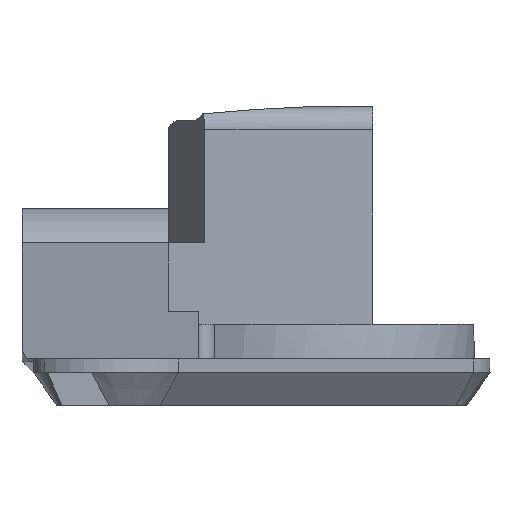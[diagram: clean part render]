
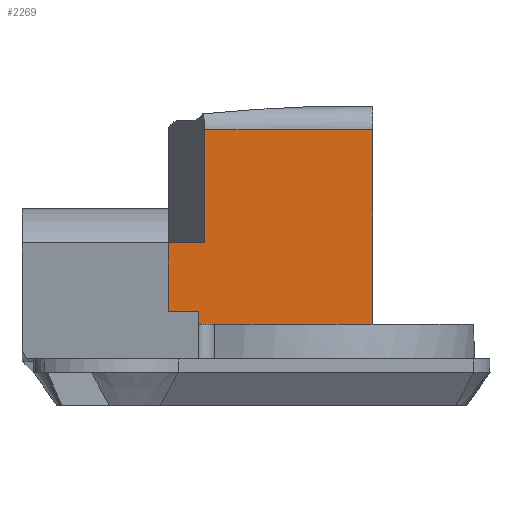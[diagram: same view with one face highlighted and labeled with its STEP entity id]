
A CAD part, left-side view. The second image highlights one B-rep face of the part: STEP entity #2269.
In plain terms, the highlighted planar face has unit normal (-1, 0, 0).
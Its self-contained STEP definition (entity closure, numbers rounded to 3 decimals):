
#254=FACE_OUTER_BOUND('',#388,.T.);
#388=EDGE_LOOP('',(#1855,#1856,#1857,#1858,#1859,#1860,#1861,#1862));
#459=LINE('',#3239,#682);
#611=LINE('',#3870,#834);
#618=LINE('',#3888,#841);
#619=LINE('',#3890,#842);
#620=LINE('',#3892,#843);
#621=LINE('',#3893,#844);
#622=LINE('',#3895,#845);
#623=LINE('',#3896,#846);
#682=VECTOR('',#2597,1000.);
#834=VECTOR('',#2965,10.);
#841=VECTOR('',#2980,10.);
#842=VECTOR('',#2981,1000.);
#843=VECTOR('',#2982,10.);
#844=VECTOR('',#2983,10.);
#845=VECTOR('',#2984,1000.);
#846=VECTOR('',#2985,1000.);
#919=VERTEX_POINT('',#3236);
#920=VERTEX_POINT('',#3238);
#1052=VERTEX_POINT('',#3867);
#1053=VERTEX_POINT('',#3869);
#1060=VERTEX_POINT('',#3887);
#1061=VERTEX_POINT('',#3889);
#1062=VERTEX_POINT('',#3891);
#1063=VERTEX_POINT('',#3894);
#1133=EDGE_CURVE('',#919,#920,#459,.T.);
#1339=EDGE_CURVE('',#1052,#1053,#611,.F.);
#1348=EDGE_CURVE('',#1060,#1052,#618,.T.);
#1349=EDGE_CURVE('',#1061,#1060,#619,.T.);
#1350=EDGE_CURVE('',#1061,#1062,#620,.T.);
#1351=EDGE_CURVE('',#1062,#920,#621,.F.);
#1352=EDGE_CURVE('',#1063,#919,#622,.T.);
#1353=EDGE_CURVE('',#1053,#1063,#623,.T.);
#1855=ORIENTED_EDGE('',*,*,#1339,.F.);
#1856=ORIENTED_EDGE('',*,*,#1348,.F.);
#1857=ORIENTED_EDGE('',*,*,#1349,.F.);
#1858=ORIENTED_EDGE('',*,*,#1350,.T.);
#1859=ORIENTED_EDGE('',*,*,#1351,.T.);
#1860=ORIENTED_EDGE('',*,*,#1133,.F.);
#1861=ORIENTED_EDGE('',*,*,#1352,.F.);
#1862=ORIENTED_EDGE('',*,*,#1353,.F.);
#2163=PLANE('',#2470);
#2269=ADVANCED_FACE('',(#254),#2163,.F.);
#2470=AXIS2_PLACEMENT_3D('',#3886,#2978,#2979);
#2597=DIRECTION('',(0.,1.,0.));
#2965=DIRECTION('',(0.,0.,1.));
#2978=DIRECTION('center_axis',(1.,0.,0.));
#2979=DIRECTION('ref_axis',(0.,0.,
-1.));
#2980=DIRECTION('',(0.,-1.,0.));
#2981=DIRECTION('',(0.,0.,1.));
#2982=DIRECTION('',(0.,1.,0.));
#2983=DIRECTION('',(0.,0.,1.));
#2984=DIRECTION('',(0.,0.,1.));
#2985=DIRECTION('',(0.,1.,0.));
#3236=CARTESIAN_POINT('',(-18.037,-1.852,-40.686));
#3238=CARTESIAN_POINT('',(-18.037,-0.552,-40.686));
#3239=CARTESIAN_POINT('',(-18.037,-12.59,-40.686));
#3867=CARTESIAN_POINT('',(-18.037,-9.37,-32.873));
#3869=CARTESIAN_POINT('',(-18.037,-9.37,-41.249));
#3870=CARTESIAN_POINT('',(-18.037,-9.37,-24.749));
#3886=CARTESIAN_POINT('Origin',(-18.037,-12.59,-26.749));
#3887=CARTESIAN_POINT('',(-18.037,-2.138,-32.873));
#3888=CARTESIAN_POINT('',(-18.037,-9.161,-32.873));
#3889=CARTESIAN_POINT('',(-18.037,-2.138,-37.749));
#3890=CARTESIAN_POINT('',(-18.037,-2.138,-26.749));
#3891=CARTESIAN_POINT('',(-18.037,-0.552,-37.749));
#3892=CARTESIAN_POINT('',(-18.037,-6.295,-37.749));
#3893=CARTESIAN_POINT('',(-18.037,-0.552,-33.999));
#3894=CARTESIAN_POINT('',(-18.037,-1.852,-41.249));
#3895=CARTESIAN_POINT('',(-18.037,-1.852,-26.749));
#3896=CARTESIAN_POINT('',(-18.037,-9.666,-41.249));
